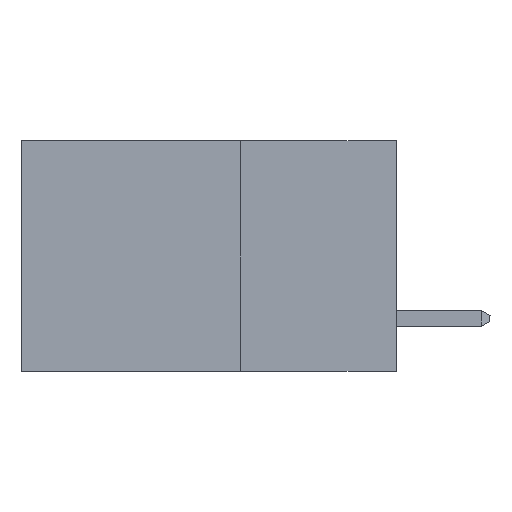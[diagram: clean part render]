
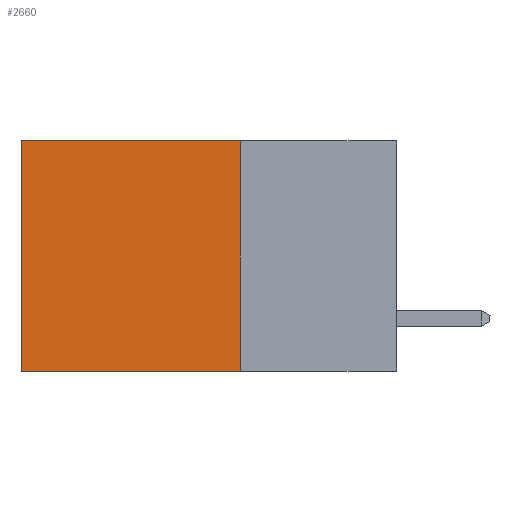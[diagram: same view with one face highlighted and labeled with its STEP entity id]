
A CAD part, left-side view. The second image highlights one B-rep face of the part: STEP entity #2660.
In plain terms, the highlighted planar face has unit normal (-1, 0, 0).
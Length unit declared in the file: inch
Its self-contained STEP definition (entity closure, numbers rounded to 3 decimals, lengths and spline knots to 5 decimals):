
#784 = LINE ( 'NONE', #9925, #11590 ) ;
#1533 = VECTOR ( 'NONE', #7566, 39.37008 ) ;
#1667 = CARTESIAN_POINT ( 'NONE',  ( 0.2615, 0.25, -0.37 ) ) ;
#1804 = CARTESIAN_POINT ( 'NONE',  ( 0.2615, 0.6, -0.37 ) ) ;
#2658 = EDGE_LOOP ( 'NONE', ( #7919, #12094, #12092, #10565 ) ) ;
#2660 = ADVANCED_FACE ( 'NONE', ( #12759 ), #4918, .F. ) ;
#3517 = CARTESIAN_POINT ( 'NONE',  ( 0.2615, 0.25, -0.37 ) ) ;
#3548 = DIRECTION ( 'NONE',  ( 0., 1., 0. ) ) ;
#3578 = DIRECTION ( 'NONE',  ( 0., 0., -1. ) ) ;
#3829 = VERTEX_POINT ( 'NONE', #15338 ) ;
#3926 = DIRECTION ( 'NONE',  ( 1., 0., 0. ) ) ;
#4918 = PLANE ( 'NONE',  #17955 ) ;
#7566 = DIRECTION ( 'NONE',  ( 0., 0., -1. ) ) ;
#7919 = ORIENTED_EDGE ( 'NONE', *, *, #17776, .T. ) ;
#9142 = LINE ( 'NONE', #1804, #1533 ) ;
#9157 = VERTEX_POINT ( 'NONE', #15295 ) ;
#9837 = DIRECTION ( 'NONE',  ( 0., 1., 0. ) ) ;
#9895 = CARTESIAN_POINT ( 'NONE',  ( 0.2615, 0.25, -0.37 ) ) ;
#9925 = CARTESIAN_POINT ( 'NONE',  ( 0.2615, 0.25, 0. ) ) ;
#10332 = LINE ( 'NONE', #3517, #17074 ) ;
#10565 = ORIENTED_EDGE ( 'NONE', *, *, #11197, .T. ) ;
#11197 = EDGE_CURVE ( 'NONE', #3829, #12955, #784, .T. ) ;
#11242 = DIRECTION ( 'NONE',  ( 0., 0., -1. ) ) ;
#11590 = VECTOR ( 'NONE', #9837, 39.37008 ) ;
#11951 = EDGE_CURVE ( 'NONE', #9157, #14714, #10332, .T. ) ;
#12092 = ORIENTED_EDGE ( 'NONE', *, *, #17597, .F. ) ;
#12094 = ORIENTED_EDGE ( 'NONE', *, *, #11951, .F. ) ;
#12113 = VECTOR ( 'NONE', #11242, 39.37008 ) ;
#12759 = FACE_OUTER_BOUND ( 'NONE', #2658, .T. ) ;
#12955 = VERTEX_POINT ( 'NONE', #14137 ) ;
#12969 = LINE ( 'NONE', #9895, #12113 ) ;
#13842 = CARTESIAN_POINT ( 'NONE',  ( 0.2615, 0.6, -0.37 ) ) ;
#14137 = CARTESIAN_POINT ( 'NONE',  ( 0.2615, 0.6, 0. ) ) ;
#14714 = VERTEX_POINT ( 'NONE', #13842 ) ;
#15295 = CARTESIAN_POINT ( 'NONE',  ( 0.2615, 0.25, -0.37 ) ) ;
#15338 = CARTESIAN_POINT ( 'NONE',  ( 0.2615, 0.25, 0. ) ) ;
#17074 = VECTOR ( 'NONE', #3548, 39.37008 ) ;
#17597 = EDGE_CURVE ( 'NONE', #3829, #9157, #12969, .T. ) ;
#17776 = EDGE_CURVE ( 'NONE', #12955, #14714, #9142, .T. ) ;
#17955 = AXIS2_PLACEMENT_3D ( 'NONE', #1667, #3926, #3578 ) ;
